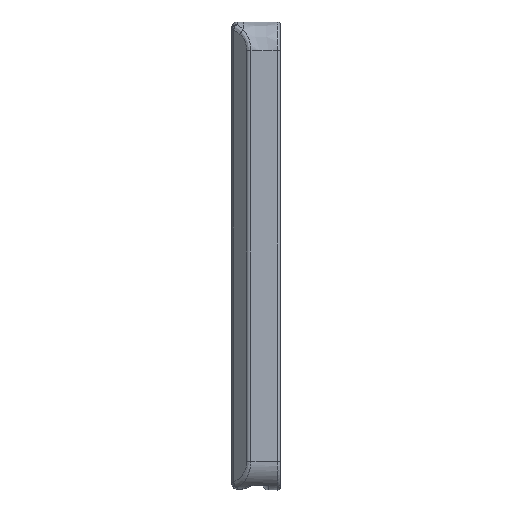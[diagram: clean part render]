
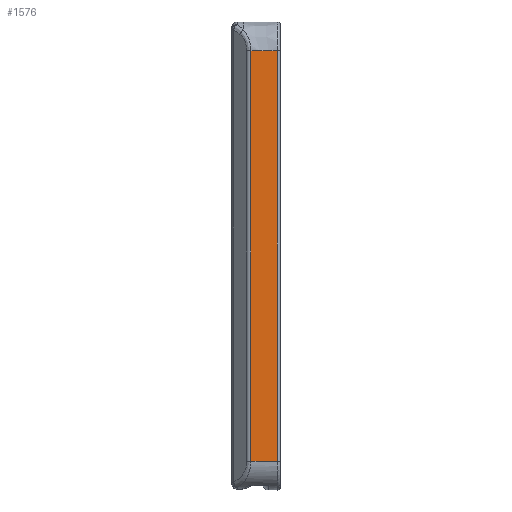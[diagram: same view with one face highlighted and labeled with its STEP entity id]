
A CAD part, left-side view. The second image highlights one B-rep face of the part: STEP entity #1576.
In plain terms, the highlighted planar face has unit normal (-1, 0, 0).
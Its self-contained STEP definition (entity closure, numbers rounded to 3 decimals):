
#15=PLANE('',#1719);
#105=LINE('',#2912,#200);
#106=LINE('',#2913,#201);
#107=LINE('',#2914,#202);
#200=VECTOR('',#1954,1000.);
#201=VECTOR('',#1955,1000.);
#202=VECTOR('',#1956,1000.);
#380=FACE_OUTER_BOUND('',#482,.T.);
#482=EDGE_LOOP('',(#1109,#1110,#1111,#1112));
#592=CIRCLE('',#1713,471.424);
#689=VERTEX_POINT('',#2511);
#690=VERTEX_POINT('',#2512);
#696=VERTEX_POINT('',#2910);
#697=VERTEX_POINT('',#2911);
#843=EDGE_CURVE('',#689,#690,#592,.T.);
#853=EDGE_CURVE('',#696,#697,#105,.T.);
#854=EDGE_CURVE('',#697,#690,#106,.T.);
#855=EDGE_CURVE('',#689,#696,#107,.T.);
#1109=ORIENTED_EDGE('',*,*,#853,.T.);
#1110=ORIENTED_EDGE('',*,*,#854,.T.);
#1111=ORIENTED_EDGE('',*,*,#843,.F.);
#1112=ORIENTED_EDGE('',*,*,#855,.T.);
#1576=ADVANCED_FACE('',(#380),#15,.T.);
#1713=AXIS2_PLACEMENT_3D('',#2513,#1940,#1941);
#1719=AXIS2_PLACEMENT_3D('',#2909,#1952,#1953);
#1940=DIRECTION('center_axis',(1.,0.,0.));
#1941=DIRECTION('ref_axis',(0.,-0.005,1.));
#1952=DIRECTION('center_axis',(-1.,0.,0.));
#1953=DIRECTION('ref_axis',(0.,-0.241,-0.97));
#1954=DIRECTION('',(0.,-1.,0.));
#1955=DIRECTION('',(0.,0.,1.));
#1956=DIRECTION('',(0.,0.,-1.));
#2511=CARTESIAN_POINT('',(-15.342,-113.346,-3.958));
#2512=CARTESIAN_POINT('',(-15.342,-117.008,-3.961));
#2513=CARTESIAN_POINT('Origin',(-15.342,-114.874,-475.38));
#2909=CARTESIAN_POINT('Origin',(-15.342,-99.907,-6.957));
#2910=CARTESIAN_POINT('',(-15.342,-113.346,-60.547));
#2911=CARTESIAN_POINT('',(-15.342,-117.008,-60.547));
#2912=CARTESIAN_POINT('',(-15.342,-113.346,-60.547));
#2913=CARTESIAN_POINT('',(-15.342,-117.008,-60.547));
#2914=CARTESIAN_POINT('',(-15.342,-113.346,-3.958));
